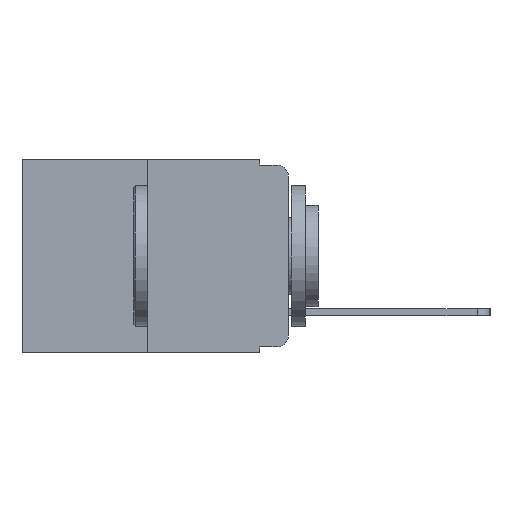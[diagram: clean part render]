
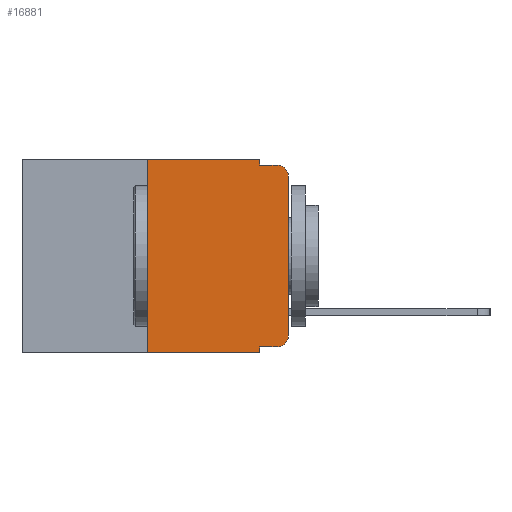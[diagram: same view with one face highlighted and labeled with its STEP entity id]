
A CAD part, left-side view. The second image highlights one B-rep face of the part: STEP entity #16881.
In plain terms, the highlighted planar face has unit normal (-1, 0, 0).
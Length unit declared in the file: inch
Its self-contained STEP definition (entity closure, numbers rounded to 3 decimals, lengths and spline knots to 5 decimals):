
#50 = CARTESIAN_POINT ( 'NONE',  ( 0., 0.25, 0. ) ) ;
#85 = CARTESIAN_POINT ( 'NONE',  ( 0., 0.051, -0.343 ) ) ;
#141 = VERTEX_POINT ( 'NONE', #9288 ) ;
#282 = VECTOR ( 'NONE', #728, 39.37008 ) ;
#728 = DIRECTION ( 'NONE',  ( 0., -1., 0. ) ) ;
#1085 = DIRECTION ( 'NONE',  ( 1., 0., 0. ) ) ;
#1227 = EDGE_CURVE ( 'NONE', #10311, #12683, #16380, .T. ) ;
#1291 = EDGE_CURVE ( 'NONE', #17242, #2940, #7726, .T. ) ;
#1604 = VERTEX_POINT ( 'NONE', #15025 ) ;
#1626 = VECTOR ( 'NONE', #9461, 39.37008 ) ;
#2284 = CARTESIAN_POINT ( 'NONE',  ( 0., 0.051, -0.333 ) ) ;
#2321 = LINE ( 'NONE', #50, #5443 ) ;
#2322 = CARTESIAN_POINT ( 'NONE',  ( 0., 0.051, 0. ) ) ;
#2651 = DIRECTION ( 'NONE',  ( 0., -1., 0. ) ) ;
#2940 = VERTEX_POINT ( 'NONE', #85 ) ;
#3278 = VECTOR ( 'NONE', #12993, 39.37008 ) ;
#3444 = CIRCLE ( 'NONE', #5145, 0.02 ) ;
#3666 = EDGE_CURVE ( 'NONE', #17242, #7025, #10468, .T. ) ;
#3699 = DIRECTION ( 'NONE',  ( 0., 0., -1. ) ) ;
#3830 = EDGE_LOOP ( 'NONE', ( #12503, #10933, #11796, #11967, #12755, #12547, #9752, #9577, #14679, #6910 ) ) ;
#3837 = CARTESIAN_POINT ( 'NONE',  ( 0., 0.051, 0. ) ) ;
#4037 = LINE ( 'NONE', #9885, #282 ) ;
#4078 = CARTESIAN_POINT ( 'NONE',  ( 0., 0.473, 0. ) ) ;
#4303 = EDGE_CURVE ( 'NONE', #7025, #13723, #3444, .T. ) ;
#4572 = DIRECTION ( 'NONE',  ( 0., -1., 0. ) ) ;
#4582 = EDGE_CURVE ( 'NONE', #1604, #11149, #2321, .T. ) ;
#4780 = DIRECTION ( 'NONE',  ( 0., 0., 1. ) ) ;
#5145 = AXIS2_PLACEMENT_3D ( 'NONE', #5686, #15948, #7210 ) ;
#5225 = DIRECTION ( 'NONE',  ( 0., 0., -1. ) ) ;
#5384 = AXIS2_PLACEMENT_3D ( 'NONE', #5832, #16093, #7377 ) ;
#5443 = VECTOR ( 'NONE', #4780, 39.37008 ) ;
#5686 = CARTESIAN_POINT ( 'NONE',  ( 0., 0.02, -0.313 ) ) ;
#5721 = FACE_OUTER_BOUND ( 'NONE', #3830, .T. ) ;
#5822 = EDGE_CURVE ( 'NONE', #11149, #10311, #18772, .T. ) ;
#5832 = CARTESIAN_POINT ( 'NONE',  ( 0., 0.02, -0.03 ) ) ;
#5949 = EDGE_CURVE ( 'NONE', #141, #12300, #19209, .T. ) ;
#6786 = CARTESIAN_POINT ( 'NONE',  ( 0., 0.25, 0. ) ) ;
#6910 = ORIENTED_EDGE ( 'NONE', *, *, #4303, .T. ) ;
#7025 = VERTEX_POINT ( 'NONE', #18546 ) ;
#7210 = DIRECTION ( 'NONE',  ( 0., 0., -1. ) ) ;
#7377 = DIRECTION ( 'NONE',  ( 0., 0., -1. ) ) ;
#7726 = LINE ( 'NONE', #3837, #18750 ) ;
#8556 = AXIS2_PLACEMENT_3D ( 'NONE', #18768, #1085, #11721 ) ;
#8743 = PLANE ( 'NONE',  #8556 ) ;
#9288 = CARTESIAN_POINT ( 'NONE',  ( 0., 0., -0.03 ) ) ;
#9461 = DIRECTION ( 'NONE',  ( 0., 0., 1. ) ) ;
#9527 = CARTESIAN_POINT ( 'NONE',  ( 0., 0., -0.313 ) ) ;
#9577 = ORIENTED_EDGE ( 'NONE', *, *, #1291, .F. ) ;
#9712 = LINE ( 'NONE', #13876, #1626 ) ;
#9752 = ORIENTED_EDGE ( 'NONE', *, *, #18684, .T. ) ;
#9885 = CARTESIAN_POINT ( 'NONE',  ( 0., 0.473, -0.343 ) ) ;
#10192 = VECTOR ( 'NONE', #2651, 39.37008 ) ;
#10311 = VERTEX_POINT ( 'NONE', #2322 ) ;
#10468 = LINE ( 'NONE', #2284, #18527 ) ;
#10933 = ORIENTED_EDGE ( 'NONE', *, *, #5949, .T. ) ;
#11149 = VERTEX_POINT ( 'NONE', #6786 ) ;
#11536 = CARTESIAN_POINT ( 'NONE',  ( 0., 0.02, -0.01 ) ) ;
#11721 = DIRECTION ( 'NONE',  ( 0., 0., -1. ) ) ;
#11796 = ORIENTED_EDGE ( 'NONE', *, *, #13413, .F. ) ;
#11967 = ORIENTED_EDGE ( 'NONE', *, *, #1227, .F. ) ;
#12300 = VERTEX_POINT ( 'NONE', #11536 ) ;
#12503 = ORIENTED_EDGE ( 'NONE', *, *, #16015, .T. ) ;
#12512 = CARTESIAN_POINT ( 'NONE',  ( 0., 0.051, -0.333 ) ) ;
#12547 = ORIENTED_EDGE ( 'NONE', *, *, #4582, .F. ) ;
#12614 = VECTOR ( 'NONE', #3699, 39.37008 ) ;
#12683 = VERTEX_POINT ( 'NONE', #15638 ) ;
#12755 = ORIENTED_EDGE ( 'NONE', *, *, #5822, .F. ) ;
#12993 = DIRECTION ( 'NONE',  ( 0., -1., 0. ) ) ;
#13413 = EDGE_CURVE ( 'NONE', #12683, #12300, #14596, .T. ) ;
#13723 = VERTEX_POINT ( 'NONE', #9527 ) ;
#13876 = CARTESIAN_POINT ( 'NONE',  ( 0., 0., 0. ) ) ;
#14590 = CARTESIAN_POINT ( 'NONE',  ( 0., 0.051, -0.01 ) ) ;
#14596 = LINE ( 'NONE', #14590, #10192 ) ;
#14679 = ORIENTED_EDGE ( 'NONE', *, *, #3666, .T. ) ;
#15025 = CARTESIAN_POINT ( 'NONE',  ( 0., 0.25, -0.343 ) ) ;
#15638 = CARTESIAN_POINT ( 'NONE',  ( 0., 0.051, -0.01 ) ) ;
#15666 = CARTESIAN_POINT ( 'NONE',  ( 0., 0.051, 0. ) ) ;
#15948 = DIRECTION ( 'NONE',  ( -1., 0., 0. ) ) ;
#16015 = EDGE_CURVE ( 'NONE', #13723, #141, #9712, .T. ) ;
#16093 = DIRECTION ( 'NONE',  ( -1., 0., 0. ) ) ;
#16380 = LINE ( 'NONE', #15666, #12614 ) ;
#16881 = ADVANCED_FACE ( 'NONE', ( #5721 ), #8743, .F. ) ;
#17242 = VERTEX_POINT ( 'NONE', #12512 ) ;
#18527 = VECTOR ( 'NONE', #4572, 39.37008 ) ;
#18546 = CARTESIAN_POINT ( 'NONE',  ( 0., 0.02, -0.333 ) ) ;
#18684 = EDGE_CURVE ( 'NONE', #1604, #2940, #4037, .T. ) ;
#18750 = VECTOR ( 'NONE', #5225, 39.37008 ) ;
#18768 = CARTESIAN_POINT ( 'NONE',  ( 0., 0.473, 0. ) ) ;
#18772 = LINE ( 'NONE', #4078, #3278 ) ;
#19209 = CIRCLE ( 'NONE', #5384, 0.02 ) ;
